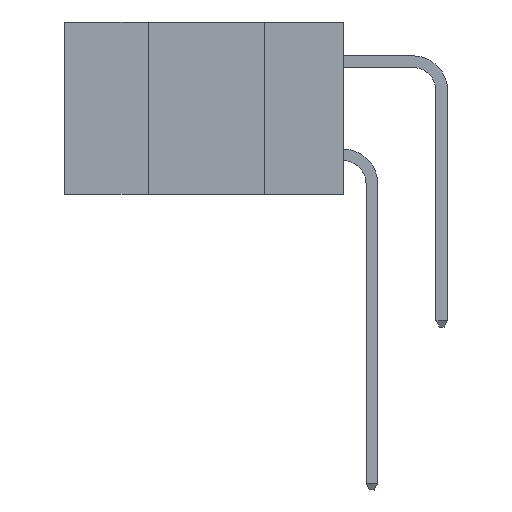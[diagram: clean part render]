
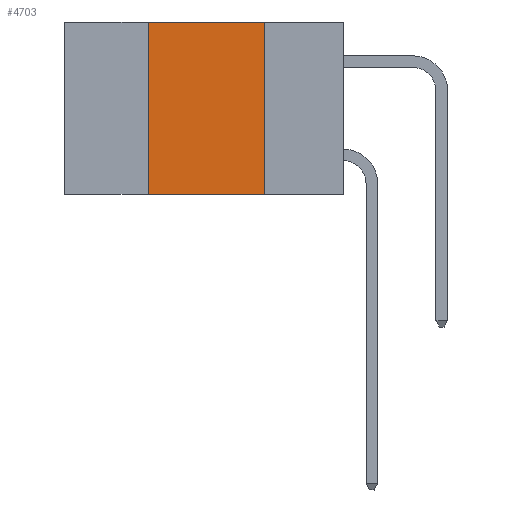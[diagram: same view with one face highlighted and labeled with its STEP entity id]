
A CAD part, left-side view. The second image highlights one B-rep face of the part: STEP entity #4703.
In plain terms, the highlighted planar face has unit normal (-1, 0, 0).
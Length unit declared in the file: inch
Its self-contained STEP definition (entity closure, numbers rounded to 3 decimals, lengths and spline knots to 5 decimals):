
#748 = CARTESIAN_POINT ( 'NONE',  ( 0., 0.17, 0. ) ) ;
#953 = ORIENTED_EDGE ( 'NONE', *, *, #1121, .F. ) ;
#1121 = EDGE_CURVE ( 'NONE', #9193, #3427, #9971, .T. ) ;
#1232 = LINE ( 'NONE', #3955, #11570 ) ;
#1673 = PLANE ( 'NONE',  #3865 ) ;
#1714 = DIRECTION ( 'NONE',  ( 1., 0., 0. ) ) ;
#1720 = EDGE_CURVE ( 'NONE', #11078, #9193, #1232, .T. ) ;
#2088 = CARTESIAN_POINT ( 'NONE',  ( 0., 0.17, 0. ) ) ;
#2758 = VECTOR ( 'NONE', #10190, 39.37008 ) ;
#3254 = VECTOR ( 'NONE', #11287, 39.37008 ) ;
#3337 = VERTEX_POINT ( 'NONE', #3535 ) ;
#3427 = VERTEX_POINT ( 'NONE', #6341 ) ;
#3439 = EDGE_LOOP ( 'NONE', ( #953, #8389, #8749, #11431 ) ) ;
#3535 = CARTESIAN_POINT ( 'NONE',  ( 0., 0.42, -0.37 ) ) ;
#3592 = LINE ( 'NONE', #12427, #5092 ) ;
#3865 = AXIS2_PLACEMENT_3D ( 'NONE', #9336, #1714, #12271 ) ;
#3955 = CARTESIAN_POINT ( 'NONE',  ( 0., 0.6, 0. ) ) ;
#4334 = CARTESIAN_POINT ( 'NONE',  ( 0., 0.6, -0.37 ) ) ;
#4703 = ADVANCED_FACE ( 'NONE', ( #10919 ), #1673, .F. ) ;
#5092 = VECTOR ( 'NONE', #7841, 39.37008 ) ;
#6039 = LINE ( 'NONE', #4334, #2758 ) ;
#6341 = CARTESIAN_POINT ( 'NONE',  ( 0., 0.17, -0.37 ) ) ;
#7841 = DIRECTION ( 'NONE',  ( 0., 0., 1. ) ) ;
#8389 = ORIENTED_EDGE ( 'NONE', *, *, #1720, .F. ) ;
#8611 = CARTESIAN_POINT ( 'NONE',  ( 0., 0.42, 0. ) ) ;
#8749 = ORIENTED_EDGE ( 'NONE', *, *, #11671, .F. ) ;
#9193 = VERTEX_POINT ( 'NONE', #2088 ) ;
#9336 = CARTESIAN_POINT ( 'NONE',  ( 0., 0.6, 0. ) ) ;
#9471 = EDGE_CURVE ( 'NONE', #3337, #3427, #6039, .T. ) ;
#9971 = LINE ( 'NONE', #748, #3254 ) ;
#10190 = DIRECTION ( 'NONE',  ( 0., -1., 0. ) ) ;
#10651 = DIRECTION ( 'NONE',  ( 0., -1., 0. ) ) ;
#10919 = FACE_OUTER_BOUND ( 'NONE', #3439, .T. ) ;
#11078 = VERTEX_POINT ( 'NONE', #8611 ) ;
#11287 = DIRECTION ( 'NONE',  ( 0., 0., -1. ) ) ;
#11431 = ORIENTED_EDGE ( 'NONE', *, *, #9471, .T. ) ;
#11570 = VECTOR ( 'NONE', #10651, 39.37008 ) ;
#11671 = EDGE_CURVE ( 'NONE', #3337, #11078, #3592, .T. ) ;
#12271 = DIRECTION ( 'NONE',  ( 0., 0., -1. ) ) ;
#12427 = CARTESIAN_POINT ( 'NONE',  ( 0., 0.42, 0. ) ) ;
